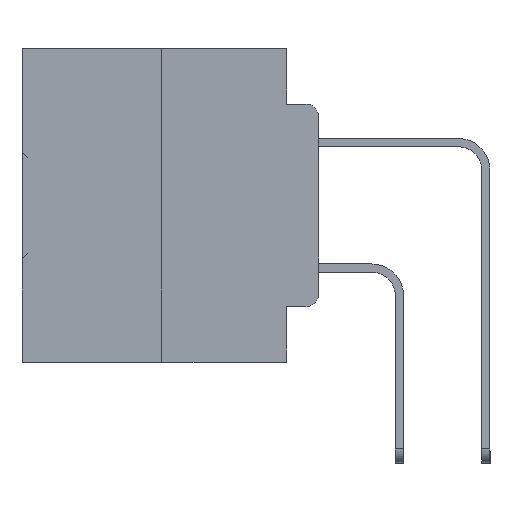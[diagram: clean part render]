
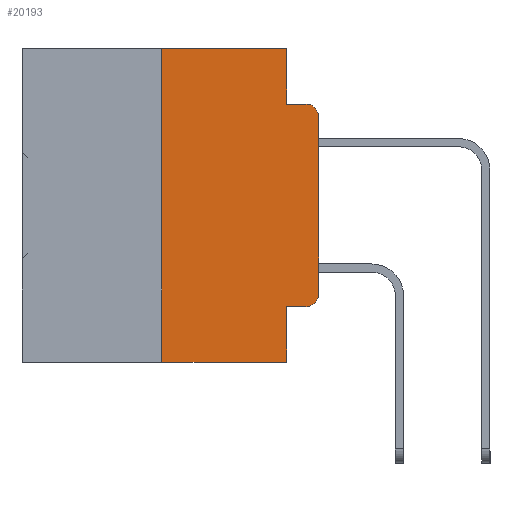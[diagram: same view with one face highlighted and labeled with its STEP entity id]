
A CAD part, left-side view. The second image highlights one B-rep face of the part: STEP entity #20193.
In plain terms, the highlighted planar face has unit normal (-1, 0, 0).
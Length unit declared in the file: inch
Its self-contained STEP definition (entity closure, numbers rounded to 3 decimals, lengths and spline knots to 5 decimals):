
#271 = AXIS2_PLACEMENT_3D ( 'NONE', #13177, #33056, #16084 ) ;
#652 = CARTESIAN_POINT ( 'NONE',  ( 0., 0.473, -0.5 ) ) ;
#2111 = CARTESIAN_POINT ( 'NONE',  ( 0., 0., -0.1085 ) ) ;
#2327 = CIRCLE ( 'NONE', #271, 0.02 ) ;
#3546 = CARTESIAN_POINT ( 'NONE',  ( 0., 0.25, 0. ) ) ;
#3897 = EDGE_CURVE ( 'NONE', #34843, #7971, #14711, .T. ) ;
#4119 = EDGE_CURVE ( 'NONE', #31172, #14065, #15149, .T. ) ;
#5157 = CARTESIAN_POINT ( 'NONE',  ( 0., 0.25, -0.5 ) ) ;
#5675 = CARTESIAN_POINT ( 'NONE',  ( 0., 0.051, -0.5 ) ) ;
#5797 = CARTESIAN_POINT ( 'NONE',  ( 0., 0.051, 0. ) ) ;
#5845 = CARTESIAN_POINT ( 'NONE',  ( 0., 0.051, -0.0885 ) ) ;
#6787 = CARTESIAN_POINT ( 'NONE',  ( 0., 0.02, -0.4115 ) ) ;
#7460 = VECTOR ( 'NONE', #35991, 39.37008 ) ;
#7971 = VERTEX_POINT ( 'NONE', #5675 ) ;
#8694 = DIRECTION ( 'NONE',  ( 0., 0., -1. ) ) ;
#9830 = CARTESIAN_POINT ( 'NONE',  ( 0., 0.02, -0.1085 ) ) ;
#9911 = EDGE_CURVE ( 'NONE', #31172, #7971, #15359, .T. ) ;
#10320 = VERTEX_POINT ( 'NONE', #2111 ) ;
#10516 = AXIS2_PLACEMENT_3D ( 'NONE', #34554, #11953, #31865 ) ;
#10842 = VECTOR ( 'NONE', #18551, 39.37008 ) ;
#10855 = EDGE_LOOP ( 'NONE', ( #14262, #23118, #35502, #27699, #12513, #24970, #28996, #13871, #26326, #22738 ) ) ;
#11061 = LINE ( 'NONE', #5845, #27152 ) ;
#11354 = DIRECTION ( 'NONE',  ( 0., -1., 0. ) ) ;
#11487 = CARTESIAN_POINT ( 'NONE',  ( 0., 0.051, -0.0885 ) ) ;
#11845 = EDGE_CURVE ( 'NONE', #34843, #19136, #15087, .T. ) ;
#11953 = DIRECTION ( 'NONE',  ( 1., 0., 0. ) ) ;
#12513 = ORIENTED_EDGE ( 'NONE', *, *, #18567, .F. ) ;
#12722 = DIRECTION ( 'NONE',  ( 0., 0., -1. ) ) ;
#13177 = CARTESIAN_POINT ( 'NONE',  ( 0., 0.02, -0.3915 ) ) ;
#13800 = EDGE_CURVE ( 'NONE', #18550, #23059, #14068, .T. ) ;
#13871 = ORIENTED_EDGE ( 'NONE', *, *, #9911, .F. ) ;
#14065 = VERTEX_POINT ( 'NONE', #6787 ) ;
#14068 = LINE ( 'NONE', #5797, #35762 ) ;
#14262 = ORIENTED_EDGE ( 'NONE', *, *, #25222, .T. ) ;
#14523 = DIRECTION ( 'NONE',  ( 0., -1., 0. ) ) ;
#14711 = LINE ( 'NONE', #652, #36396 ) ;
#15087 = LINE ( 'NONE', #16236, #7460 ) ;
#15119 = CARTESIAN_POINT ( 'NONE',  ( 0., 0., -0.3915 ) ) ;
#15149 = LINE ( 'NONE', #19734, #29374 ) ;
#15238 = VERTEX_POINT ( 'NONE', #15119 ) ;
#15359 = LINE ( 'NONE', #31742, #29580 ) ;
#15481 = CIRCLE ( 'NONE', #22539, 0.02 ) ;
#15677 = CARTESIAN_POINT ( 'NONE',  ( 0., 0.473, 0. ) ) ;
#15709 = CARTESIAN_POINT ( 'NONE',  ( 0., 0.051, -0.4115 ) ) ;
#16084 = DIRECTION ( 'NONE',  ( 0., 0., -1. ) ) ;
#16236 = CARTESIAN_POINT ( 'NONE',  ( 0., 0.25, 0. ) ) ;
#18438 = CARTESIAN_POINT ( 'NONE',  ( 0., 0.051, 0. ) ) ;
#18520 = DIRECTION ( 'NONE',  ( 0., 0., 1. ) ) ;
#18550 = VERTEX_POINT ( 'NONE', #18438 ) ;
#18551 = DIRECTION ( 'NONE',  ( 0., -1., 0. ) ) ;
#18567 = EDGE_CURVE ( 'NONE', #19136, #18550, #34404, .T. ) ;
#19136 = VERTEX_POINT ( 'NONE', #3546 ) ;
#19734 = CARTESIAN_POINT ( 'NONE',  ( 0., 0.051, -0.4115 ) ) ;
#20193 = ADVANCED_FACE ( 'NONE', ( #31196 ), #28901, .F. ) ;
#21432 = EDGE_CURVE ( 'NONE', #23059, #31079, #11061, .T. ) ;
#22539 = AXIS2_PLACEMENT_3D ( 'NONE', #9830, #29778, #12722 ) ;
#22715 = LINE ( 'NONE', #32624, #29386 ) ;
#22738 = ORIENTED_EDGE ( 'NONE', *, *, #35385, .T. ) ;
#23059 = VERTEX_POINT ( 'NONE', #11487 ) ;
#23118 = ORIENTED_EDGE ( 'NONE', *, *, #23304, .T. ) ;
#23304 = EDGE_CURVE ( 'NONE', #10320, #31079, #15481, .T. ) ;
#24850 = DIRECTION ( 'NONE',  ( 0., -1., 0. ) ) ;
#24970 = ORIENTED_EDGE ( 'NONE', *, *, #11845, .F. ) ;
#25222 = EDGE_CURVE ( 'NONE', #15238, #10320, #22715, .T. ) ;
#26166 = DIRECTION ( 'NONE',  ( 0., 0., -1. ) ) ;
#26326 = ORIENTED_EDGE ( 'NONE', *, *, #4119, .T. ) ;
#27152 = VECTOR ( 'NONE', #14523, 39.37008 ) ;
#27699 = ORIENTED_EDGE ( 'NONE', *, *, #13800, .F. ) ;
#28901 = PLANE ( 'NONE',  #10516 ) ;
#28996 = ORIENTED_EDGE ( 'NONE', *, *, #3897, .T. ) ;
#29374 = VECTOR ( 'NONE', #24850, 39.37008 ) ;
#29386 = VECTOR ( 'NONE', #18520, 39.37008 ) ;
#29580 = VECTOR ( 'NONE', #26166, 39.37008 ) ;
#29778 = DIRECTION ( 'NONE',  ( -1., 0., 0. ) ) ;
#31079 = VERTEX_POINT ( 'NONE', #35252 ) ;
#31172 = VERTEX_POINT ( 'NONE', #15709 ) ;
#31196 = FACE_OUTER_BOUND ( 'NONE', #10855, .T. ) ;
#31742 = CARTESIAN_POINT ( 'NONE',  ( 0., 0.051, 0. ) ) ;
#31865 = DIRECTION ( 'NONE',  ( 0., 0., -1. ) ) ;
#32624 = CARTESIAN_POINT ( 'NONE',  ( 0., 0., 0. ) ) ;
#33056 = DIRECTION ( 'NONE',  ( -1., 0., 0. ) ) ;
#34404 = LINE ( 'NONE', #15677, #10842 ) ;
#34554 = CARTESIAN_POINT ( 'NONE',  ( 0., 0.473, 0. ) ) ;
#34843 = VERTEX_POINT ( 'NONE', #5157 ) ;
#35252 = CARTESIAN_POINT ( 'NONE',  ( 0., 0.02, -0.0885 ) ) ;
#35385 = EDGE_CURVE ( 'NONE', #14065, #15238, #2327, .T. ) ;
#35502 = ORIENTED_EDGE ( 'NONE', *, *, #21432, .F. ) ;
#35762 = VECTOR ( 'NONE', #8694, 39.37008 ) ;
#35991 = DIRECTION ( 'NONE',  ( 0., 0., 1. ) ) ;
#36396 = VECTOR ( 'NONE', #11354, 39.37008 ) ;
